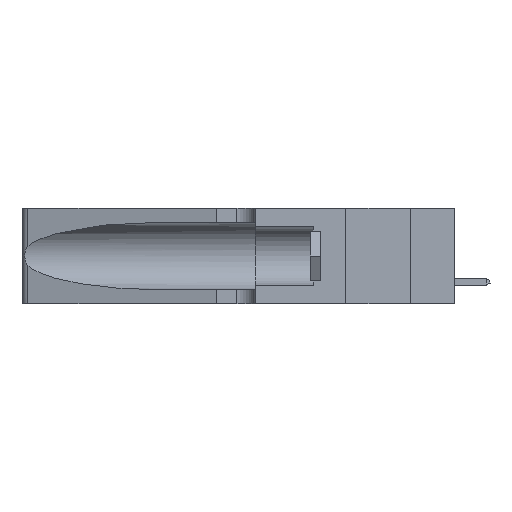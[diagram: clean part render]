
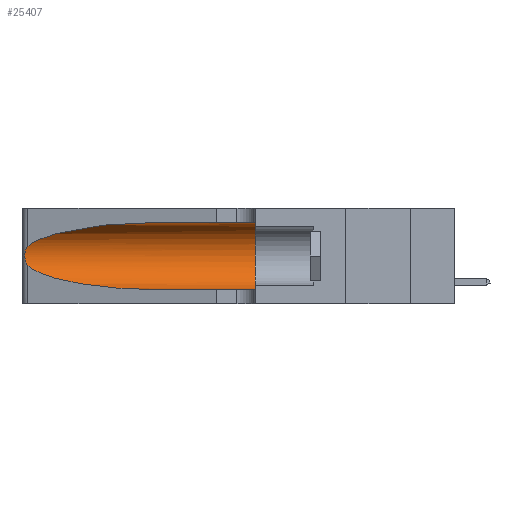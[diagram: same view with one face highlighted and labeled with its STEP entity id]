
A CAD part, left-side view. The second image highlights one B-rep face of the part: STEP entity #25407.
In plain terms, the highlighted cylindrical face has radius 3.308 mm (diameter 6.617 mm), a partial arc.
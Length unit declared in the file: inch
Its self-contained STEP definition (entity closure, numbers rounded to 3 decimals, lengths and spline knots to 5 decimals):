
#10 = CARTESIAN_POINT ( 'NONE',  ( 0.1305, 0.72297, 0.31525 ) ) ;
#38 = CARTESIAN_POINT ( 'NONE',  ( 0.25639, 1.23186, 0.15144 ) ) ;
#579 = CARTESIAN_POINT ( 'NONE',  ( 0.25487, 1.22718, 0.14631 ) ) ;
#632 = CARTESIAN_POINT ( 'NONE',  ( 0.1305, 0.72297, 0.31525 ) ) ;
#982 = CARTESIAN_POINT ( 'NONE',  ( 0.1305, 0.35, 0.31525 ) ) ;
#1038 = FACE_OUTER_BOUND ( 'NONE', #23854, .T. ) ;
#1813 = CYLINDRICAL_SURFACE ( 'NONE', #4595, 0.13025 ) ;
#2029 = EDGE_CURVE ( 'NONE', #8526, #19214, #22880, .T. ) ;
#2157 = CARTESIAN_POINT ( 'NONE',  ( 0.1305, 0.72297, 0.05475 ) ) ;
#2265 = CARTESIAN_POINT ( 'NONE',  ( 0.25854, 1.2359, 0.20912 ) ) ;
#2357 =( BOUNDED_CURVE ( )  B_SPLINE_CURVE ( 3, ( #632, #20111, #17647, #5686 ),
 .UNSPECIFIED., .F., .F. ) 
 B_SPLINE_CURVE_WITH_KNOTS ( ( 4, 4 ),
 ( 1.5708, 2.84003 ),
 .UNSPECIFIED. ) 
 CURVE ( )  GEOMETRIC_REPRESENTATION_ITEM ( )  RATIONAL_B_SPLINE_CURVE ( ( 1., 0.87, 0.87, 1. ) ) 
 REPRESENTATION_ITEM ( '' )  );
#2565 = CARTESIAN_POINT ( 'NONE',  ( 0.26075, 1.23896, 0.19203 ) ) ;
#2668 = CARTESIAN_POINT ( 'NONE',  ( 0.25555, 1.22994, 0.2215 ) ) ;
#3292 = EDGE_CURVE ( 'NONE', #25421, #11522, #2357, .T. ) ;
#3333 = DIRECTION ( 'NONE',  ( 0., 1., 0. ) ) ;
#3654 = LINE ( 'NONE', #23825, #30203 ) ;
#4026 = CARTESIAN_POINT ( 'NONE',  ( 0.25487, 1.22718, 0.14631 ) ) ;
#4595 = AXIS2_PLACEMENT_3D ( 'NONE', #4911, #28855, #7353 ) ;
#4911 = CARTESIAN_POINT ( 'NONE',  ( 0.1305, 1.61858, 0.185 ) ) ;
#4947 = CARTESIAN_POINT ( 'NONE',  ( 0.25789, 1.23486, 0.15765 ) ) ;
#5686 = CARTESIAN_POINT ( 'NONE',  ( 0.25487, 1.22718, 0.22369 ) ) ;
#5804 = CARTESIAN_POINT ( 'NONE',  ( 0.1305, 0.35, 0.185 ) ) ;
#5980 = ORIENTED_EDGE ( 'NONE', *, *, #2029, .F. ) ;
#7043 = ORIENTED_EDGE ( 'NONE', *, *, #29673, .F. ) ;
#7353 = DIRECTION ( 'NONE',  ( 0., 0., -1. ) ) ;
#7463 =( BOUNDED_CURVE ( )  B_SPLINE_CURVE ( 3, ( #579, #12918, #7974, #22406 ),
 .UNSPECIFIED., .F., .F. ) 
 B_SPLINE_CURVE_WITH_KNOTS ( ( 4, 4 ),
 ( 3.44316, 4.71239 ),
 .UNSPECIFIED. ) 
 CURVE ( )  GEOMETRIC_REPRESENTATION_ITEM ( )  RATIONAL_B_SPLINE_CURVE ( ( 1., 0.87, 0.87, 1. ) ) 
 REPRESENTATION_ITEM ( '' )  );
#7974 = CARTESIAN_POINT ( 'NONE',  ( 0.18966, 0.96281, 0.05475 ) ) ;
#8170 = EDGE_CURVE ( 'NONE', #26979, #19214, #28485, .T. ) ;
#8196 = CARTESIAN_POINT ( 'NONE',  ( 0.1305, 0.35, 0.05475 ) ) ;
#8526 = VERTEX_POINT ( 'NONE', #982 ) ;
#9720 = CARTESIAN_POINT ( 'NONE',  ( 0.25487, 1.22718, 0.14631 ) ) ;
#9933 = CARTESIAN_POINT ( 'NONE',  ( 0.26018, 1.23835, 0.19895 ) ) ;
#11522 = VERTEX_POINT ( 'NONE', #24693 ) ;
#12918 = CARTESIAN_POINT ( 'NONE',  ( 0.2373, 1.15595, 0.08982 ) ) ;
#14236 = DIRECTION ( 'NONE',  ( 0., -1., 0. ) ) ;
#14338 = VERTEX_POINT ( 'NONE', #4026 ) ;
#14793 = CARTESIAN_POINT ( 'NONE',  ( 0.25639, 1.23184, 0.21858 ) ) ;
#15280 = DIRECTION ( 'NONE',  ( 0., -1., 0. ) ) ;
#16221 = ORIENTED_EDGE ( 'NONE', *, *, #26594, .T. ) ;
#16575 = CARTESIAN_POINT ( 'NONE',  ( 0.1305, 1.61858, 0.05475 ) ) ;
#16833 = CARTESIAN_POINT ( 'NONE',  ( 0.25787, 1.23484, 0.2124 ) ) ;
#17647 = CARTESIAN_POINT ( 'NONE',  ( 0.2373, 1.15595, 0.28018 ) ) ;
#17760 = ORIENTED_EDGE ( 'NONE', *, *, #3292, .T. ) ;
#18273 = VECTOR ( 'NONE', #15280, 39.37008 ) ;
#18991 = ORIENTED_EDGE ( 'NONE', *, *, #8170, .T. ) ;
#19214 = VERTEX_POINT ( 'NONE', #8196 ) ;
#19294 = CARTESIAN_POINT ( 'NONE',  ( 0.26075, 1.23896, 0.178 ) ) ;
#19707 = CARTESIAN_POINT ( 'NONE',  ( 0.26017, 1.23833, 0.17102 ) ) ;
#20111 = CARTESIAN_POINT ( 'NONE',  ( 0.18966, 0.96281, 0.31525 ) ) ;
#21740 = CARTESIAN_POINT ( 'NONE',  ( 0.25487, 1.22718, 0.22369 ) ) ;
#22406 = CARTESIAN_POINT ( 'NONE',  ( 0.1305, 0.72297, 0.05475 ) ) ;
#22443 = AXIS2_PLACEMENT_3D ( 'NONE', #5804, #3333, #25174 ) ;
#22858 = EDGE_CURVE ( 'NONE', #11522, #14338, #23999, .T. ) ;
#22880 = CIRCLE ( 'NONE', #22443, 0.13025 ) ;
#23825 = CARTESIAN_POINT ( 'NONE',  ( 0.1305, 1.61858, 0.31525 ) ) ;
#23854 = EDGE_LOOP ( 'NONE', ( #17760, #28605, #16221, #18991, #5980, #7043 ) ) ;
#23999 = B_SPLINE_CURVE_WITH_KNOTS ( 'NONE', 3,
 ( #21740, #2668, #14793, #16833, #2265, #9933, #2565, #19294, #19707, #24347, #4947, #38, #24256, #9720 ),
 .UNSPECIFIED., .F., .F.,
 ( 4, 2, 2, 2, 2, 2, 4 ),
 ( 0., 0.00027, 0.00053, 0.00107, 0.0016, 0.00187, 0.00214 ),
 .UNSPECIFIED. ) ;
#24256 = CARTESIAN_POINT ( 'NONE',  ( 0.25555, 1.22993, 0.14849 ) ) ;
#24347 = CARTESIAN_POINT ( 'NONE',  ( 0.25856, 1.23593, 0.16098 ) ) ;
#24693 = CARTESIAN_POINT ( 'NONE',  ( 0.25487, 1.22718, 0.22369 ) ) ;
#25174 = DIRECTION ( 'NONE',  ( 0., 0., 1. ) ) ;
#25407 = ADVANCED_FACE ( 'NONE', ( #1038 ), #1813, .F. ) ;
#25421 = VERTEX_POINT ( 'NONE', #10 ) ;
#26594 = EDGE_CURVE ( 'NONE', #14338, #26979, #7463, .T. ) ;
#26979 = VERTEX_POINT ( 'NONE', #2157 ) ;
#28485 = LINE ( 'NONE', #16575, #18273 ) ;
#28605 = ORIENTED_EDGE ( 'NONE', *, *, #22858, .T. ) ;
#28855 = DIRECTION ( 'NONE',  ( 0., -1., 0. ) ) ;
#29673 = EDGE_CURVE ( 'NONE', #25421, #8526, #3654, .T. ) ;
#30203 = VECTOR ( 'NONE', #14236, 39.37008 ) ;
